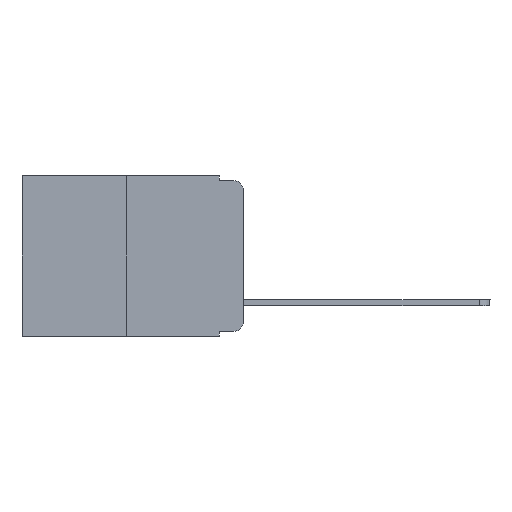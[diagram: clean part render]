
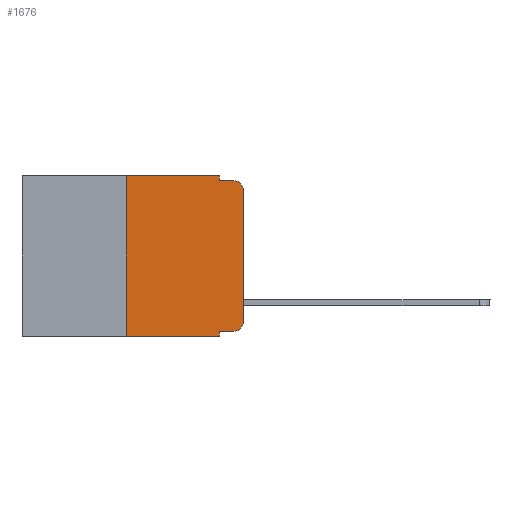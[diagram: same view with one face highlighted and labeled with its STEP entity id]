
A CAD part, left-side view. The second image highlights one B-rep face of the part: STEP entity #1676.
In plain terms, the highlighted planar face has unit normal (-1, 0, 0).
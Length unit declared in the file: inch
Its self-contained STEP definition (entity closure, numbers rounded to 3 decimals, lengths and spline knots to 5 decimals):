
#67 = LINE ( 'NONE', #5458, #5965 ) ;
#358 = DIRECTION ( 'NONE',  ( -1., 0., 0. ) ) ;
#384 = EDGE_CURVE ( 'NONE', #10801, #562, #5225, .T. ) ;
#465 = CARTESIAN_POINT ( 'NONE',  ( 0., 0.02, -0.03 ) ) ;
#562 = VERTEX_POINT ( 'NONE', #5621 ) ;
#799 = ORIENTED_EDGE ( 'NONE', *, *, #2203, .F. ) ;
#852 = LINE ( 'NONE', #2652, #4277 ) ;
#1185 = ORIENTED_EDGE ( 'NONE', *, *, #6224, .F. ) ;
#1223 = DIRECTION ( 'NONE',  ( 1., 0., 0. ) ) ;
#1226 = CARTESIAN_POINT ( 'NONE',  ( 0., 0., -0.313 ) ) ;
#1394 = ORIENTED_EDGE ( 'NONE', *, *, #5214, .T. ) ;
#1410 = VERTEX_POINT ( 'NONE', #4806 ) ;
#1524 = VECTOR ( 'NONE', #11687, 39.37008 ) ;
#1644 = ORIENTED_EDGE ( 'NONE', *, *, #6361, .T. ) ;
#1676 = ADVANCED_FACE ( 'NONE', ( #9386 ), #9563, .F. ) ;
#2113 = ORIENTED_EDGE ( 'NONE', *, *, #384, .T. ) ;
#2151 = LINE ( 'NONE', #7687, #3900 ) ;
#2203 = EDGE_CURVE ( 'NONE', #9896, #5975, #67, .T. ) ;
#2652 = CARTESIAN_POINT ( 'NONE',  ( 0., 0.051, -0.01 ) ) ;
#2746 = VECTOR ( 'NONE', #7773, 39.37008 ) ;
#2832 = DIRECTION ( 'NONE',  ( 0., 0., 1. ) ) ;
#2938 = VERTEX_POINT ( 'NONE', #6015 ) ;
#2980 = ORIENTED_EDGE ( 'NONE', *, *, #3958, .F. ) ;
#3005 = VECTOR ( 'NONE', #10674, 39.37008 ) ;
#3655 = AXIS2_PLACEMENT_3D ( 'NONE', #9502, #1223, #8616 ) ;
#3900 = VECTOR ( 'NONE', #9581, 39.37008 ) ;
#3958 = EDGE_CURVE ( 'NONE', #11465, #2938, #9167, .T. ) ;
#4277 = VECTOR ( 'NONE', #8122, 39.37008 ) ;
#4320 = CARTESIAN_POINT ( 'NONE',  ( 0., 0., 0. ) ) ;
#4352 = CIRCLE ( 'NONE', #5860, 0.02 ) ;
#4552 = DIRECTION ( 'NONE',  ( 0., -1., 0. ) ) ;
#4612 = DIRECTION ( 'NONE',  ( -1., 0., 0. ) ) ;
#4671 = AXIS2_PLACEMENT_3D ( 'NONE', #465, #358, #6759 ) ;
#4782 = EDGE_LOOP ( 'NONE', ( #2113, #1644, #1185, #6100, #2980, #10088, #6735, #799, #6527, #1394 ) ) ;
#4806 = CARTESIAN_POINT ( 'NONE',  ( 0., 0.051, -0.01 ) ) ;
#5214 = EDGE_CURVE ( 'NONE', #7171, #10801, #4352, .T. ) ;
#5225 = LINE ( 'NONE', #4320, #3005 ) ;
#5398 = DIRECTION ( 'NONE',  ( 0., 0., -1. ) ) ;
#5439 = VECTOR ( 'NONE', #2832, 39.37008 ) ;
#5458 = CARTESIAN_POINT ( 'NONE',  ( 0., 0.051, 0. ) ) ;
#5507 = CARTESIAN_POINT ( 'NONE',  ( 0., 0.473, 0. ) ) ;
#5510 = CARTESIAN_POINT ( 'NONE',  ( 0., 0.02, -0.313 ) ) ;
#5621 = CARTESIAN_POINT ( 'NONE',  ( 0., 0., -0.03 ) ) ;
#5860 = AXIS2_PLACEMENT_3D ( 'NONE', #5510, #4612, #7346 ) ;
#5965 = VECTOR ( 'NONE', #5398, 39.37008 ) ;
#5975 = VERTEX_POINT ( 'NONE', #6666 ) ;
#6015 = CARTESIAN_POINT ( 'NONE',  ( 0., 0.051, 0. ) ) ;
#6100 = ORIENTED_EDGE ( 'NONE', *, *, #6153, .F. ) ;
#6153 = EDGE_CURVE ( 'NONE', #2938, #1410, #7896, .T. ) ;
#6197 = CIRCLE ( 'NONE', #4671, 0.02 ) ;
#6224 = EDGE_CURVE ( 'NONE', #1410, #10307, #852, .T. ) ;
#6361 = EDGE_CURVE ( 'NONE', #562, #10307, #6197, .T. ) ;
#6442 = EDGE_CURVE ( 'NONE', #9896, #7171, #2151, .T. ) ;
#6527 = ORIENTED_EDGE ( 'NONE', *, *, #6442, .T. ) ;
#6666 = CARTESIAN_POINT ( 'NONE',  ( 0., 0.051, -0.343 ) ) ;
#6718 = VECTOR ( 'NONE', #4552, 39.37008 ) ;
#6735 = ORIENTED_EDGE ( 'NONE', *, *, #7598, .T. ) ;
#6759 = DIRECTION ( 'NONE',  ( 0., 0., -1. ) ) ;
#6965 = LINE ( 'NONE', #7250, #5439 ) ;
#7171 = VERTEX_POINT ( 'NONE', #11759 ) ;
#7250 = CARTESIAN_POINT ( 'NONE',  ( 0., 0.25, 0. ) ) ;
#7303 = CARTESIAN_POINT ( 'NONE',  ( 0., 0.473, -0.343 ) ) ;
#7346 = DIRECTION ( 'NONE',  ( 0., 0., -1. ) ) ;
#7598 = EDGE_CURVE ( 'NONE', #9499, #5975, #8062, .T. ) ;
#7687 = CARTESIAN_POINT ( 'NONE',  ( 0., 0.051, -0.333 ) ) ;
#7773 = DIRECTION ( 'NONE',  ( 0., 0., -1. ) ) ;
#7896 = LINE ( 'NONE', #11501, #2746 ) ;
#8062 = LINE ( 'NONE', #7303, #1524 ) ;
#8122 = DIRECTION ( 'NONE',  ( 0., -1., 0. ) ) ;
#8255 = CARTESIAN_POINT ( 'NONE',  ( 0., 0.051, -0.333 ) ) ;
#8616 = DIRECTION ( 'NONE',  ( 0., 0., -1. ) ) ;
#8882 = EDGE_CURVE ( 'NONE', #9499, #11465, #6965, .T. ) ;
#9167 = LINE ( 'NONE', #5507, #6718 ) ;
#9386 = FACE_OUTER_BOUND ( 'NONE', #4782, .T. ) ;
#9468 = CARTESIAN_POINT ( 'NONE',  ( 0., 0.25, -0.343 ) ) ;
#9499 = VERTEX_POINT ( 'NONE', #9468 ) ;
#9502 = CARTESIAN_POINT ( 'NONE',  ( 0., 0.473, 0. ) ) ;
#9563 = PLANE ( 'NONE',  #3655 ) ;
#9581 = DIRECTION ( 'NONE',  ( 0., -1., 0. ) ) ;
#9896 = VERTEX_POINT ( 'NONE', #8255 ) ;
#10088 = ORIENTED_EDGE ( 'NONE', *, *, #8882, .F. ) ;
#10163 = CARTESIAN_POINT ( 'NONE',  ( 0., 0.02, -0.01 ) ) ;
#10307 = VERTEX_POINT ( 'NONE', #10163 ) ;
#10674 = DIRECTION ( 'NONE',  ( 0., 0., 1. ) ) ;
#10801 = VERTEX_POINT ( 'NONE', #1226 ) ;
#11465 = VERTEX_POINT ( 'NONE', #11742 ) ;
#11501 = CARTESIAN_POINT ( 'NONE',  ( 0., 0.051, 0. ) ) ;
#11687 = DIRECTION ( 'NONE',  ( 0., -1., 0. ) ) ;
#11742 = CARTESIAN_POINT ( 'NONE',  ( 0., 0.25, 0. ) ) ;
#11759 = CARTESIAN_POINT ( 'NONE',  ( 0., 0.02, -0.333 ) ) ;
